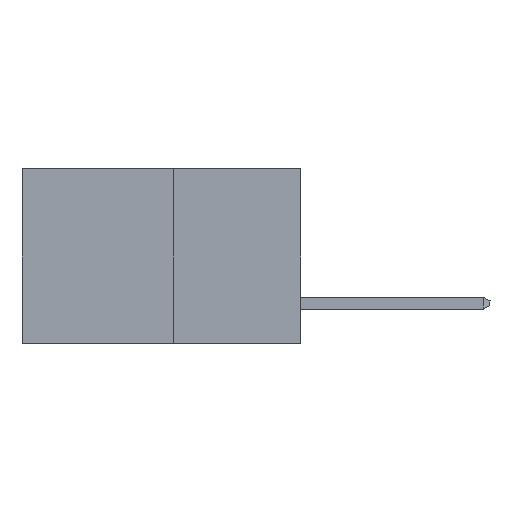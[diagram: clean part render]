
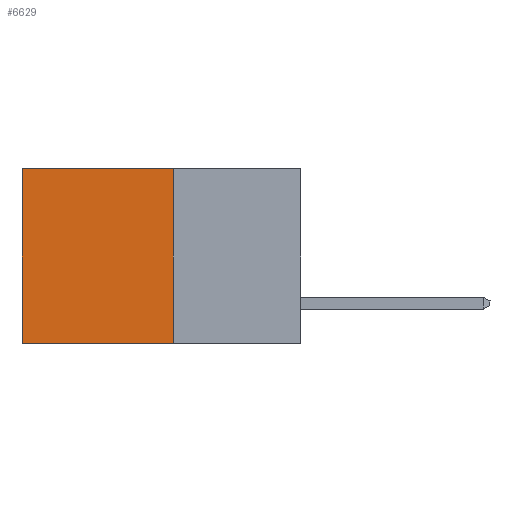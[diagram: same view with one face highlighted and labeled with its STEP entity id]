
A CAD part, left-side view. The second image highlights one B-rep face of the part: STEP entity #6629.
In plain terms, the highlighted planar face has unit normal (-1, 0, 0).
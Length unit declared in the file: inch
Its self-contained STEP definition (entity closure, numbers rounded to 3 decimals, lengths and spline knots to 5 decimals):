
#495 = CARTESIAN_POINT ( 'NONE',  ( 0.277, 0.27, -0.37 ) ) ;
#500 = VECTOR ( 'NONE', #11474, 39.37008 ) ;
#891 = LINE ( 'NONE', #11554, #500 ) ;
#2150 = VERTEX_POINT ( 'NONE', #7772 ) ;
#3414 = CARTESIAN_POINT ( 'NONE',  ( 0.277, 0.59, -0.37 ) ) ;
#3800 = EDGE_CURVE ( 'NONE', #2150, #15030, #4821, .T. ) ;
#3906 = CARTESIAN_POINT ( 'NONE',  ( 0.277, 0.27, -0.37 ) ) ;
#4396 = VERTEX_POINT ( 'NONE', #495 ) ;
#4518 = DIRECTION ( 'NONE',  ( 0., 0., -1. ) ) ;
#4821 = LINE ( 'NONE', #3414, #11382 ) ;
#4824 = VECTOR ( 'NONE', #10794, 39.37008 ) ;
#4932 = CARTESIAN_POINT ( 'NONE',  ( 0.277, 0.27, -0.37 ) ) ;
#5034 = EDGE_CURVE ( 'NONE', #9046, #2150, #891, .T. ) ;
#5230 = CARTESIAN_POINT ( 'NONE',  ( 0.277, 0.59, -0.37 ) ) ;
#5606 = ORIENTED_EDGE ( 'NONE', *, *, #3800, .T. ) ;
#5629 = CARTESIAN_POINT ( 'NONE',  ( 0.277, 0.27, -0.37 ) ) ;
#6136 = DIRECTION ( 'NONE',  ( 1., 0., 0. ) ) ;
#6629 = ADVANCED_FACE ( 'NONE', ( #12883 ), #8450, .F. ) ;
#7498 = LINE ( 'NONE', #5629, #7891 ) ;
#7772 = CARTESIAN_POINT ( 'NONE',  ( 0.277, 0.59, 0. ) ) ;
#7891 = VECTOR ( 'NONE', #14861, 39.37008 ) ;
#7989 = LINE ( 'NONE', #3906, #4824 ) ;
#8450 = PLANE ( 'NONE',  #13609 ) ;
#8653 = EDGE_LOOP ( 'NONE', ( #5606, #8718, #14767, #15107 ) ) ;
#8718 = ORIENTED_EDGE ( 'NONE', *, *, #14962, .F. ) ;
#9046 = VERTEX_POINT ( 'NONE', #14669 ) ;
#10794 = DIRECTION ( 'NONE',  ( 0., 1., 0. ) ) ;
#11382 = VECTOR ( 'NONE', #4518, 39.37008 ) ;
#11474 = DIRECTION ( 'NONE',  ( 0., 1., 0. ) ) ;
#11554 = CARTESIAN_POINT ( 'NONE',  ( 0.277, 0.27, 0. ) ) ;
#11708 = EDGE_CURVE ( 'NONE', #9046, #4396, #7498, .T. ) ;
#12883 = FACE_OUTER_BOUND ( 'NONE', #8653, .T. ) ;
#13609 = AXIS2_PLACEMENT_3D ( 'NONE', #4932, #6136, #14154 ) ;
#14154 = DIRECTION ( 'NONE',  ( 0., 0., -1. ) ) ;
#14669 = CARTESIAN_POINT ( 'NONE',  ( 0.277, 0.27, 0. ) ) ;
#14767 = ORIENTED_EDGE ( 'NONE', *, *, #11708, .F. ) ;
#14861 = DIRECTION ( 'NONE',  ( 0., 0., -1. ) ) ;
#14962 = EDGE_CURVE ( 'NONE', #4396, #15030, #7989, .T. ) ;
#15030 = VERTEX_POINT ( 'NONE', #5230 ) ;
#15107 = ORIENTED_EDGE ( 'NONE', *, *, #5034, .T. ) ;
